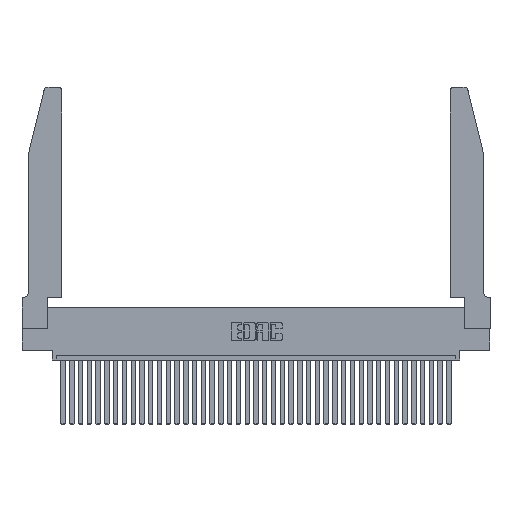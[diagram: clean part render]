
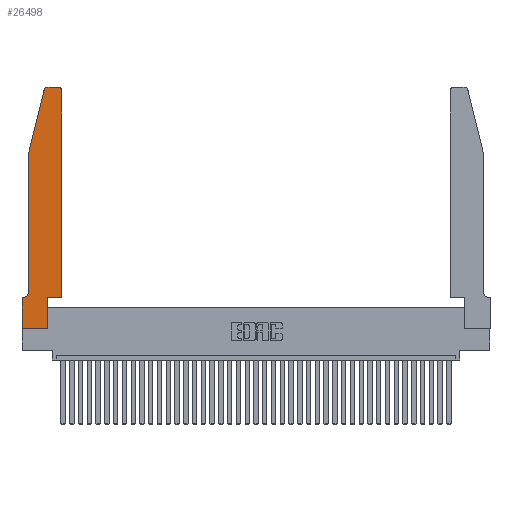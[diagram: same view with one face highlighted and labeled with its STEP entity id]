
A CAD part, top view. The second image highlights one B-rep face of the part: STEP entity #26498.
In plain terms, the highlighted planar face has unit normal (0, 0, 1).
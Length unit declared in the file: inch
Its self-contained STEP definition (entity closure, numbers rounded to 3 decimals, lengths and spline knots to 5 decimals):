
#86 = VECTOR ( 'NONE', #33775, 39.37008 ) ;
#90 = CIRCLE ( 'NONE', #15105, 0.03 ) ;
#481 = EDGE_CURVE ( 'NONE', #2488, #8281, #23487, .T. ) ;
#561 = CARTESIAN_POINT ( 'NONE',  ( 0.2865, 0., 0.37 ) ) ;
#1287 = LINE ( 'NONE', #35999, #24772 ) ;
#1410 = DIRECTION ( 'NONE',  ( 1., 0., 0. ) ) ;
#1852 = LINE ( 'NONE', #17989, #32256 ) ;
#1923 = VERTEX_POINT ( 'NONE', #20959 ) ;
#2061 = CARTESIAN_POINT ( 'NONE',  ( 0.4505, 0.35, 0.37 ) ) ;
#2301 = ORIENTED_EDGE ( 'NONE', *, *, #27121, .T. ) ;
#2488 = VERTEX_POINT ( 'NONE', #21791 ) ;
#3316 = EDGE_CURVE ( 'NONE', #31292, #26202, #20925, .T. ) ;
#4164 = VERTEX_POINT ( 'NONE', #14169 ) ;
#4342 = VERTEX_POINT ( 'NONE', #37546 ) ;
#4633 = CARTESIAN_POINT ( 'NONE',  ( 0., 0., 0.37 ) ) ;
#4732 = DIRECTION ( 'NONE',  ( 1., 0., 0. ) ) ;
#6651 = CARTESIAN_POINT ( 'NONE',  ( 0.0755, 2., 0.37 ) ) ;
#7503 = CARTESIAN_POINT ( 'NONE',  ( 0.0055, 0.42, 0.37 ) ) ;
#7510 = DIRECTION ( 'NONE',  ( -1., 0., 0. ) ) ;
#7690 = VECTOR ( 'NONE', #33925, 39.37008 ) ;
#7754 = DIRECTION ( 'NONE',  ( -1., 0., 0. ) ) ;
#8281 = VERTEX_POINT ( 'NONE', #37547 ) ;
#8339 = ORIENTED_EDGE ( 'NONE', *, *, #28677, .T. ) ;
#9983 = VERTEX_POINT ( 'NONE', #34667 ) ;
#10252 = AXIS2_PLACEMENT_3D ( 'NONE', #19819, #25385, #31727 ) ;
#10563 = ORIENTED_EDGE ( 'NONE', *, *, #17265, .T. ) ;
#11376 = ORIENTED_EDGE ( 'NONE', *, *, #34044, .T. ) ;
#11551 = VERTEX_POINT ( 'NONE', #27540 ) ;
#11607 = ORIENTED_EDGE ( 'NONE', *, *, #37304, .T. ) ;
#12191 = ORIENTED_EDGE ( 'NONE', *, *, #12645, .T. ) ;
#12550 = CIRCLE ( 'NONE', #32602, 0.07 ) ;
#12645 = EDGE_CURVE ( 'NONE', #11551, #9983, #16493, .T. ) ;
#12962 = CARTESIAN_POINT ( 'NONE',  ( 0.284, 2.75, 0.37 ) ) ;
#13330 = CARTESIAN_POINT ( 'NONE',  ( 0., 0., 0.37 ) ) ;
#13397 = EDGE_CURVE ( 'NONE', #9983, #4164, #17387, .T. ) ;
#14169 = CARTESIAN_POINT ( 'NONE',  ( 0., 0., 0.37 ) ) ;
#14535 = VECTOR ( 'NONE', #1410, 39.37008 ) ;
#14669 = CIRCLE ( 'NONE', #10252, 0.03 ) ;
#14729 = DIRECTION ( 'NONE',  ( 0., 0., 1. ) ) ;
#14848 = PLANE ( 'NONE',  #29252 ) ;
#14986 = DIRECTION ( 'NONE',  ( 1., 0., 0. ) ) ;
#15066 = CARTESIAN_POINT ( 'NONE',  ( 0.4205, 2.75, 0.37 ) ) ;
#15105 = AXIS2_PLACEMENT_3D ( 'NONE', #15188, #32995, #18156 ) ;
#15130 = DIRECTION ( 'NONE',  ( 0., 1., 0. ) ) ;
#15188 = CARTESIAN_POINT ( 'NONE',  ( 0.4205, 2.72, 0.37 ) ) ;
#15283 = ORIENTED_EDGE ( 'NONE', *, *, #37334, .T. ) ;
#15488 = DIRECTION ( 'NONE',  ( 0., -1., 0. ) ) ;
#16493 = LINE ( 'NONE', #31330, #24811 ) ;
#17265 = EDGE_CURVE ( 'NONE', #8281, #1923, #1852, .T. ) ;
#17387 = LINE ( 'NONE', #13330, #7690 ) ;
#17989 = CARTESIAN_POINT ( 'NONE',  ( 0.4505, 0.35, 0.37 ) ) ;
#18156 = DIRECTION ( 'NONE',  ( 1., 0., 0. ) ) ;
#18201 = DIRECTION ( 'NONE',  ( -0.239, -0.971, 0. ) ) ;
#18932 = CARTESIAN_POINT ( 'NONE',  ( 0.2865, 0.35, 0.37 ) ) ;
#19552 = DIRECTION ( 'NONE',  ( -1., 0., 0. ) ) ;
#19819 = CARTESIAN_POINT ( 'NONE',  ( 0.284, 2.72, 0.37 ) ) ;
#20616 = LINE ( 'NONE', #6651, #35412 ) ;
#20925 = LINE ( 'NONE', #34180, #23283 ) ;
#20959 = CARTESIAN_POINT ( 'NONE',  ( 0.4505, 2.72, 0.37 ) ) ;
#21260 = LINE ( 'NONE', #18932, #86 ) ;
#21791 = CARTESIAN_POINT ( 'NONE',  ( 0.2865, 0.35, 0.37 ) ) ;
#23283 = VECTOR ( 'NONE', #7510, 39.37008 ) ;
#23487 = LINE ( 'NONE', #2061, #24868 ) ;
#24129 = CARTESIAN_POINT ( 'NONE',  ( 0., 0.35, 0.37 ) ) ;
#24772 = VECTOR ( 'NONE', #18201, 39.37008 ) ;
#24811 = VECTOR ( 'NONE', #19552, 39.37008 ) ;
#24868 = VECTOR ( 'NONE', #4732, 39.37008 ) ;
#25027 = ORIENTED_EDGE ( 'NONE', *, *, #30968, .T. ) ;
#25385 = DIRECTION ( 'NONE',  ( 0., 0., 1. ) ) ;
#25397 = DIRECTION ( 'NONE',  ( 0., 0., -1. ) ) ;
#25490 = ORIENTED_EDGE ( 'NONE', *, *, #34794, .T. ) ;
#26202 = VERTEX_POINT ( 'NONE', #12962 ) ;
#26498 = ADVANCED_FACE ( 'NONE', ( #31497 ), #14848, .T. ) ;
#27063 = ORIENTED_EDGE ( 'NONE', *, *, #3316, .T. ) ;
#27121 = EDGE_CURVE ( 'NONE', #1923, #31292, #90, .T. ) ;
#27540 = CARTESIAN_POINT ( 'NONE',  ( 0.0055, 0.35, 0.37 ) ) ;
#28429 = ORIENTED_EDGE ( 'NONE', *, *, #13397, .T. ) ;
#28677 = EDGE_CURVE ( 'NONE', #26202, #34995, #14669, .T. ) ;
#29252 = AXIS2_PLACEMENT_3D ( 'NONE', #24129, #14729, #14986 ) ;
#30968 = EDGE_CURVE ( 'NONE', #4164, #37277, #34384, .T. ) ;
#31105 = EDGE_LOOP ( 'NONE', ( #27063, #8339, #11607, #15283, #11376, #12191, #28429, #25027, #25490, #33781, #10563, #2301 ) ) ;
#31292 = VERTEX_POINT ( 'NONE', #15066 ) ;
#31330 = CARTESIAN_POINT ( 'NONE',  ( 0.0755, 0.35, 0.37 ) ) ;
#31497 = FACE_OUTER_BOUND ( 'NONE', #31105, .T. ) ;
#31727 = DIRECTION ( 'NONE',  ( 1., 0., 0. ) ) ;
#32256 = VECTOR ( 'NONE', #15130, 39.37008 ) ;
#32602 = AXIS2_PLACEMENT_3D ( 'NONE', #7503, #25397, #7754 ) ;
#32975 = VERTEX_POINT ( 'NONE', #34659 ) ;
#32995 = DIRECTION ( 'NONE',  ( 0., 0., 1. ) ) ;
#33775 = DIRECTION ( 'NONE',  ( 0., 1., 0. ) ) ;
#33781 = ORIENTED_EDGE ( 'NONE', *, *, #481, .T. ) ;
#33925 = DIRECTION ( 'NONE',  ( 0., -1., 0. ) ) ;
#34044 = EDGE_CURVE ( 'NONE', #4342, #11551, #12550, .T. ) ;
#34180 = CARTESIAN_POINT ( 'NONE',  ( 0.2605, 2.75, 0.37 ) ) ;
#34384 = LINE ( 'NONE', #4633, #14535 ) ;
#34659 = CARTESIAN_POINT ( 'NONE',  ( 0.0755, 2., 0.37 ) ) ;
#34667 = CARTESIAN_POINT ( 'NONE',  ( 0., 0.35, 0.37 ) ) ;
#34794 = EDGE_CURVE ( 'NONE', #37277, #2488, #21260, .T. ) ;
#34816 = CARTESIAN_POINT ( 'NONE',  ( 0.25487, 2.72718, 0.37 ) ) ;
#34995 = VERTEX_POINT ( 'NONE', #34816 ) ;
#35412 = VECTOR ( 'NONE', #15488, 39.37008 ) ;
#35999 = CARTESIAN_POINT ( 'NONE',  ( 0.0755, 2., 0.37 ) ) ;
#37277 = VERTEX_POINT ( 'NONE', #561 ) ;
#37304 = EDGE_CURVE ( 'NONE', #34995, #32975, #1287, .T. ) ;
#37334 = EDGE_CURVE ( 'NONE', #32975, #4342, #20616, .T. ) ;
#37546 = CARTESIAN_POINT ( 'NONE',  ( 0.0755, 0.42, 0.37 ) ) ;
#37547 = CARTESIAN_POINT ( 'NONE',  ( 0.4505, 0.35, 0.37 ) ) ;
